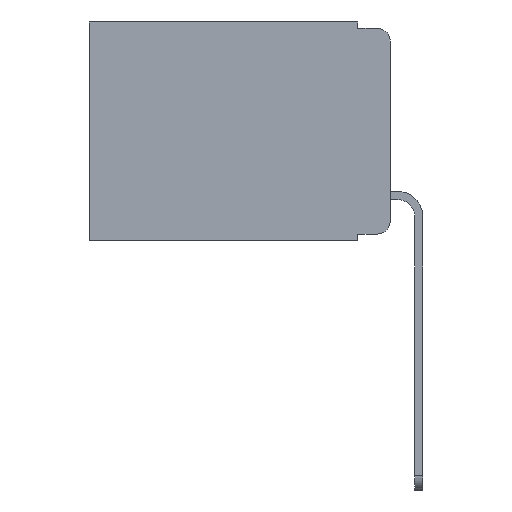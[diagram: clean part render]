
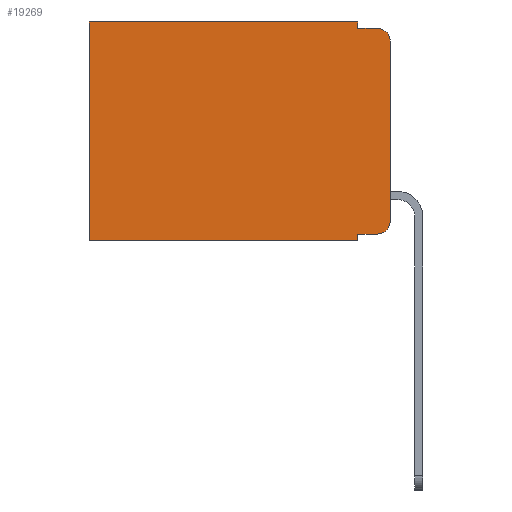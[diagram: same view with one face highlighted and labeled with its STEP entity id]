
A CAD part, left-side view. The second image highlights one B-rep face of the part: STEP entity #19269.
In plain terms, the highlighted planar face has unit normal (-1, 0, 0).
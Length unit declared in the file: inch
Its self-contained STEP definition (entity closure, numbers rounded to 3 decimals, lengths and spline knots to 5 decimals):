
#621 = VECTOR ( 'NONE', #5011, 39.37008 ) ;
#674 = VECTOR ( 'NONE', #2708, 39.37008 ) ;
#1287 = CARTESIAN_POINT ( 'NONE',  ( 0.298, 0., 0. ) ) ;
#1321 = EDGE_CURVE ( 'NONE', #11775, #5547, #10072, .T. ) ;
#1371 = FACE_OUTER_BOUND ( 'NONE', #18676, .T. ) ;
#1404 = CARTESIAN_POINT ( 'NONE',  ( 0.298, 0.051, -0.01 ) ) ;
#1503 = VERTEX_POINT ( 'NONE', #19558 ) ;
#1613 = VERTEX_POINT ( 'NONE', #4194 ) ;
#2333 = CARTESIAN_POINT ( 'NONE',  ( 0.298, 0., -0.313 ) ) ;
#2346 = EDGE_CURVE ( 'NONE', #8788, #11775, #5979, .T. ) ;
#2708 = DIRECTION ( 'NONE',  ( 0., 0., -1. ) ) ;
#2748 = VECTOR ( 'NONE', #6006, 39.37008 ) ;
#2903 = DIRECTION ( 'NONE',  ( 0., 0., -1. ) ) ;
#3251 = VERTEX_POINT ( 'NONE', #14020 ) ;
#4194 = CARTESIAN_POINT ( 'NONE',  ( 0.298, 0.051, -0.343 ) ) ;
#4535 = EDGE_CURVE ( 'NONE', #1613, #5547, #11800, .T. ) ;
#4691 = CARTESIAN_POINT ( 'NONE',  ( 0.298, 0.473, -0.343 ) ) ;
#4901 = EDGE_CURVE ( 'NONE', #8788, #6912, #12992, .T. ) ;
#5011 = DIRECTION ( 'NONE',  ( 0., 1., 0. ) ) ;
#5530 = ORIENTED_EDGE ( 'NONE', *, *, #4901, .F. ) ;
#5534 = DIRECTION ( 'NONE',  ( 0., 0., -1. ) ) ;
#5547 = VERTEX_POINT ( 'NONE', #4691 ) ;
#5977 = ORIENTED_EDGE ( 'NONE', *, *, #19011, .F. ) ;
#5979 = LINE ( 'NONE', #12462, #8349 ) ;
#6006 = DIRECTION ( 'NONE',  ( 0., -1., 0. ) ) ;
#6415 = VECTOR ( 'NONE', #8187, 39.37008 ) ;
#6798 = LINE ( 'NONE', #1404, #2748 ) ;
#6912 = VERTEX_POINT ( 'NONE', #14760 ) ;
#6977 = DIRECTION ( 'NONE',  ( 0., 0., -1. ) ) ;
#7304 = VERTEX_POINT ( 'NONE', #17117 ) ;
#8187 = DIRECTION ( 'NONE',  ( 0., -1., 0. ) ) ;
#8349 = VECTOR ( 'NONE', #9330, 39.37008 ) ;
#8583 = PLANE ( 'NONE',  #18318 ) ;
#8788 = VERTEX_POINT ( 'NONE', #10673 ) ;
#9245 = ORIENTED_EDGE ( 'NONE', *, *, #1321, .T. ) ;
#9330 = DIRECTION ( 'NONE',  ( 0., 1., 0. ) ) ;
#9367 = CARTESIAN_POINT ( 'NONE',  ( 0.298, 0.051, -0.333 ) ) ;
#9380 = EDGE_CURVE ( 'NONE', #1503, #7304, #11111, .T. ) ;
#9608 = ORIENTED_EDGE ( 'NONE', *, *, #9380, .T. ) ;
#9633 = CARTESIAN_POINT ( 'NONE',  ( 0.298, 0., -0.343 ) ) ;
#10072 = LINE ( 'NONE', #11990, #18432 ) ;
#10388 = EDGE_CURVE ( 'NONE', #6912, #7304, #6798, .T. ) ;
#10612 = CARTESIAN_POINT ( 'NONE',  ( 0.298, 0.473, 0. ) ) ;
#10672 = CARTESIAN_POINT ( 'NONE',  ( 0.298, 0.051, 0. ) ) ;
#10673 = CARTESIAN_POINT ( 'NONE',  ( 0.298, 0.051, 0. ) ) ;
#11111 = CIRCLE ( 'NONE', #16741, 0.02 ) ;
#11495 = ORIENTED_EDGE ( 'NONE', *, *, #10388, .F. ) ;
#11775 = VERTEX_POINT ( 'NONE', #10612 ) ;
#11800 = LINE ( 'NONE', #9633, #621 ) ;
#11924 = DIRECTION ( 'NONE',  ( 0., 0., -1. ) ) ;
#11990 = CARTESIAN_POINT ( 'NONE',  ( 0.298, 0.473, 0. ) ) ;
#12390 = AXIS2_PLACEMENT_3D ( 'NONE', #18823, #12775, #16016 ) ;
#12462 = CARTESIAN_POINT ( 'NONE',  ( 0.298, 0., 0. ) ) ;
#12762 = EDGE_CURVE ( 'NONE', #3251, #17858, #15470, .T. ) ;
#12775 = DIRECTION ( 'NONE',  ( -1., 0., 0. ) ) ;
#12807 = DIRECTION ( 'NONE',  ( -1., 0., 0. ) ) ;
#12992 = LINE ( 'NONE', #10672, #16526 ) ;
#13116 = CARTESIAN_POINT ( 'NONE',  ( 0.298, 0., 0. ) ) ;
#13165 = VERTEX_POINT ( 'NONE', #9367 ) ;
#13522 = ORIENTED_EDGE ( 'NONE', *, *, #4535, .F. ) ;
#13859 = CARTESIAN_POINT ( 'NONE',  ( 0.298, 0.051, -0.333 ) ) ;
#14020 = CARTESIAN_POINT ( 'NONE',  ( 0.298, 0.02, -0.333 ) ) ;
#14597 = ORIENTED_EDGE ( 'NONE', *, *, #19120, .T. ) ;
#14627 = DIRECTION ( 'NONE',  ( 1., 0., 0. ) ) ;
#14760 = CARTESIAN_POINT ( 'NONE',  ( 0.298, 0.051, -0.01 ) ) ;
#15330 = ORIENTED_EDGE ( 'NONE', *, *, #16989, .F. ) ;
#15470 = CIRCLE ( 'NONE', #12390, 0.02 ) ;
#15978 = CARTESIAN_POINT ( 'NONE',  ( 0.298, 0.02, -0.03 ) ) ;
#16016 = DIRECTION ( 'NONE',  ( 0., 0., -1. ) ) ;
#16436 = CARTESIAN_POINT ( 'NONE',  ( 0.298, 0.051, 0. ) ) ;
#16526 = VECTOR ( 'NONE', #16588, 39.37008 ) ;
#16588 = DIRECTION ( 'NONE',  ( 0., 0., -1. ) ) ;
#16741 = AXIS2_PLACEMENT_3D ( 'NONE', #15978, #12807, #6977 ) ;
#16805 = ORIENTED_EDGE ( 'NONE', *, *, #12762, .T. ) ;
#16810 = LINE ( 'NONE', #16436, #674 ) ;
#16989 = EDGE_CURVE ( 'NONE', #13165, #1613, #16810, .T. ) ;
#17117 = CARTESIAN_POINT ( 'NONE',  ( 0.298, 0.02, -0.01 ) ) ;
#17858 = VERTEX_POINT ( 'NONE', #2333 ) ;
#18318 = AXIS2_PLACEMENT_3D ( 'NONE', #13116, #14627, #5534 ) ;
#18416 = ORIENTED_EDGE ( 'NONE', *, *, #2346, .T. ) ;
#18432 = VECTOR ( 'NONE', #2903, 39.37008 ) ;
#18525 = LINE ( 'NONE', #1287, #19226 ) ;
#18676 = EDGE_LOOP ( 'NONE', ( #5977, #9608, #11495, #5530, #18416, #9245, #13522, #15330, #14597, #16805 ) ) ;
#18823 = CARTESIAN_POINT ( 'NONE',  ( 0.298, 0.02, -0.313 ) ) ;
#19007 = LINE ( 'NONE', #13859, #6415 ) ;
#19011 = EDGE_CURVE ( 'NONE', #1503, #17858, #18525, .T. ) ;
#19120 = EDGE_CURVE ( 'NONE', #13165, #3251, #19007, .T. ) ;
#19226 = VECTOR ( 'NONE', #11924, 39.37008 ) ;
#19269 = ADVANCED_FACE ( 'NONE', ( #1371 ), #8583, .F. ) ;
#19558 = CARTESIAN_POINT ( 'NONE',  ( 0.298, 0., -0.03 ) ) ;
